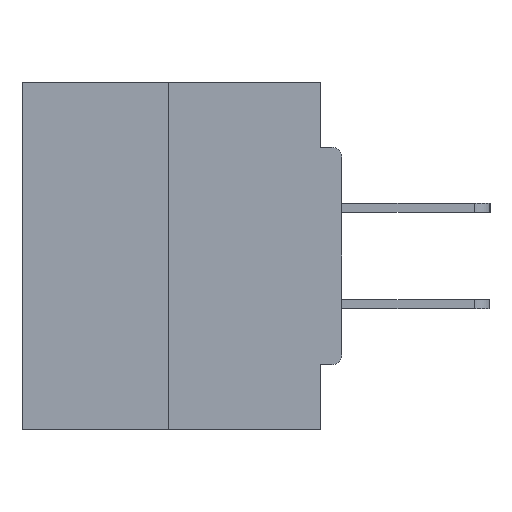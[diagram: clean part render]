
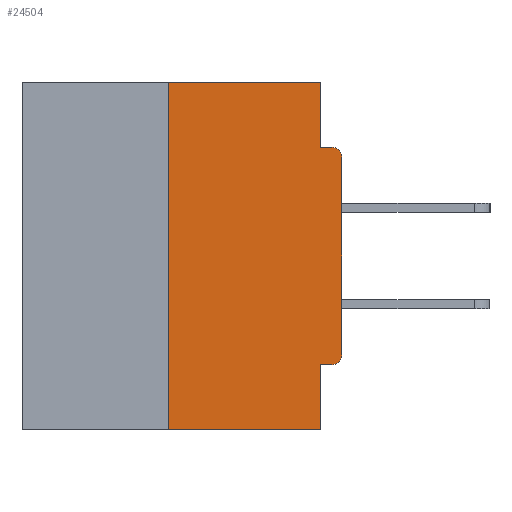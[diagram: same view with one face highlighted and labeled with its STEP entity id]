
A CAD part, left-side view. The second image highlights one B-rep face of the part: STEP entity #24504.
In plain terms, the highlighted planar face has unit normal (-1, 0, 0).
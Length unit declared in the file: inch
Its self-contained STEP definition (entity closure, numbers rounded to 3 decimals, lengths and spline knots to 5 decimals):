
#153 = LINE ( 'NONE', #21160, #10408 ) ;
#1027 = PLANE ( 'NONE',  #7817 ) ;
#1333 = CARTESIAN_POINT ( 'NONE',  ( 0., 0.031, -0.5 ) ) ;
#1667 = CIRCLE ( 'NONE', #7021, 0.015 ) ;
#2076 = CARTESIAN_POINT ( 'NONE',  ( 0., 0.25, -0.5 ) ) ;
#3086 = CARTESIAN_POINT ( 'NONE',  ( 0., 0., -0.3915 ) ) ;
#3103 = LINE ( 'NONE', #10801, #29433 ) ;
#3773 = ORIENTED_EDGE ( 'NONE', *, *, #5209, .T. ) ;
#3821 = CARTESIAN_POINT ( 'NONE',  ( 0., 0.46, 0. ) ) ;
#3864 = VECTOR ( 'NONE', #13528, 39.37008 ) ;
#5209 = EDGE_CURVE ( 'NONE', #28884, #12042, #21963, .T. ) ;
#6161 = LINE ( 'NONE', #11346, #18301 ) ;
#6567 = DIRECTION ( 'NONE',  ( 1., 0., 0. ) ) ;
#6850 = DIRECTION ( 'NONE',  ( 0., 0., -1. ) ) ;
#7021 = AXIS2_PLACEMENT_3D ( 'NONE', #30451, #27894, #24156 ) ;
#7236 = EDGE_LOOP ( 'NONE', ( #30805, #23453, #16780, #24602, #28934, #11545, #13261, #3773, #13718, #27101 ) ) ;
#7817 = AXIS2_PLACEMENT_3D ( 'NONE', #26764, #6567, #11266 ) ;
#7933 = VERTEX_POINT ( 'NONE', #22407 ) ;
#7979 = VERTEX_POINT ( 'NONE', #12443 ) ;
#8024 = CARTESIAN_POINT ( 'NONE',  ( 0., 0., -0.4065 ) ) ;
#8767 = DIRECTION ( 'NONE',  ( 0., -1., 0. ) ) ;
#9161 = EDGE_CURVE ( 'NONE', #17962, #7979, #15578, .T. ) ;
#9647 = CARTESIAN_POINT ( 'NONE',  ( 0., 0.015, -0.0935 ) ) ;
#10387 = VERTEX_POINT ( 'NONE', #16504 ) ;
#10408 = VECTOR ( 'NONE', #16284, 39.37008 ) ;
#10801 = CARTESIAN_POINT ( 'NONE',  ( 0., 0., 0. ) ) ;
#10902 = VECTOR ( 'NONE', #25854, 39.37008 ) ;
#11266 = DIRECTION ( 'NONE',  ( 0., 0., -1. ) ) ;
#11346 = CARTESIAN_POINT ( 'NONE',  ( 0., 0.031, -0.5 ) ) ;
#11534 = LINE ( 'NONE', #32125, #31478 ) ;
#11545 = ORIENTED_EDGE ( 'NONE', *, *, #21106, .T. ) ;
#11548 = EDGE_CURVE ( 'NONE', #10387, #7933, #11534, .T. ) ;
#12042 = VERTEX_POINT ( 'NONE', #9647 ) ;
#12443 = CARTESIAN_POINT ( 'NONE',  ( 0., 0.031, -0.4065 ) ) ;
#12738 = CARTESIAN_POINT ( 'NONE',  ( 0., 0.015, -0.4065 ) ) ;
#13010 = EDGE_CURVE ( 'NONE', #28650, #28884, #3103, .T. ) ;
#13261 = ORIENTED_EDGE ( 'NONE', *, *, #13010, .T. ) ;
#13321 = VERTEX_POINT ( 'NONE', #2076 ) ;
#13507 = CARTESIAN_POINT ( 'NONE',  ( 0., 0.25, 0. ) ) ;
#13528 = DIRECTION ( 'NONE',  ( 0., -1., 0. ) ) ;
#13718 = ORIENTED_EDGE ( 'NONE', *, *, #33293, .F. ) ;
#14375 = CARTESIAN_POINT ( 'NONE',  ( 0., 0.25, 0. ) ) ;
#15298 = CARTESIAN_POINT ( 'NONE',  ( 0., 0., -0.1085 ) ) ;
#15515 = AXIS2_PLACEMENT_3D ( 'NONE', #21858, #30284, #27744 ) ;
#15578 = LINE ( 'NONE', #8024, #10902 ) ;
#15834 = EDGE_CURVE ( 'NONE', #22573, #10387, #23640, .T. ) ;
#16058 = LINE ( 'NONE', #13507, #25382 ) ;
#16284 = DIRECTION ( 'NONE',  ( 0., -1., 0. ) ) ;
#16504 = CARTESIAN_POINT ( 'NONE',  ( 0., 0.031, 0. ) ) ;
#16667 = LINE ( 'NONE', #26276, #20945 ) ;
#16780 = ORIENTED_EDGE ( 'NONE', *, *, #27586, .T. ) ;
#17962 = VERTEX_POINT ( 'NONE', #12738 ) ;
#18301 = VECTOR ( 'NONE', #18614, 39.37008 ) ;
#18614 = DIRECTION ( 'NONE',  ( 0., 0., -1. ) ) ;
#20945 = VECTOR ( 'NONE', #8767, 39.37008 ) ;
#21073 = DIRECTION ( 'NONE',  ( 0., 0., 1. ) ) ;
#21106 = EDGE_CURVE ( 'NONE', #17962, #28650, #1667, .T. ) ;
#21150 = EDGE_CURVE ( 'NONE', #7979, #28185, #6161, .T. ) ;
#21160 = CARTESIAN_POINT ( 'NONE',  ( 0., 0., -0.0935 ) ) ;
#21858 = CARTESIAN_POINT ( 'NONE',  ( 0., 0.015, -0.1085 ) ) ;
#21963 = CIRCLE ( 'NONE', #15515, 0.015 ) ;
#22407 = CARTESIAN_POINT ( 'NONE',  ( 0., 0.031, -0.0935 ) ) ;
#22573 = VERTEX_POINT ( 'NONE', #14375 ) ;
#23453 = ORIENTED_EDGE ( 'NONE', *, *, #29966, .F. ) ;
#23640 = LINE ( 'NONE', #3821, #3864 ) ;
#24156 = DIRECTION ( 'NONE',  ( 0., 0., -1. ) ) ;
#24504 = ADVANCED_FACE ( 'NONE', ( #29651 ), #1027, .F. ) ;
#24602 = ORIENTED_EDGE ( 'NONE', *, *, #21150, .F. ) ;
#25382 = VECTOR ( 'NONE', #28873, 39.37008 ) ;
#25854 = DIRECTION ( 'NONE',  ( 0., 1., 0. ) ) ;
#26276 = CARTESIAN_POINT ( 'NONE',  ( 0., 0.46, -0.5 ) ) ;
#26764 = CARTESIAN_POINT ( 'NONE',  ( 0., 0.46, 0. ) ) ;
#27101 = ORIENTED_EDGE ( 'NONE', *, *, #11548, .F. ) ;
#27586 = EDGE_CURVE ( 'NONE', #13321, #28185, #16667, .T. ) ;
#27744 = DIRECTION ( 'NONE',  ( 0., 0., -1. ) ) ;
#27894 = DIRECTION ( 'NONE',  ( -1., 0., 0. ) ) ;
#28185 = VERTEX_POINT ( 'NONE', #1333 ) ;
#28650 = VERTEX_POINT ( 'NONE', #3086 ) ;
#28873 = DIRECTION ( 'NONE',  ( 0., 0., 1. ) ) ;
#28884 = VERTEX_POINT ( 'NONE', #15298 ) ;
#28934 = ORIENTED_EDGE ( 'NONE', *, *, #9161, .F. ) ;
#29433 = VECTOR ( 'NONE', #21073, 39.37008 ) ;
#29651 = FACE_OUTER_BOUND ( 'NONE', #7236, .T. ) ;
#29966 = EDGE_CURVE ( 'NONE', #13321, #22573, #16058, .T. ) ;
#30284 = DIRECTION ( 'NONE',  ( -1., 0., 0. ) ) ;
#30451 = CARTESIAN_POINT ( 'NONE',  ( 0., 0.015, -0.3915 ) ) ;
#30805 = ORIENTED_EDGE ( 'NONE', *, *, #15834, .F. ) ;
#31478 = VECTOR ( 'NONE', #6850, 39.37008 ) ;
#32125 = CARTESIAN_POINT ( 'NONE',  ( 0., 0.031, 0. ) ) ;
#33293 = EDGE_CURVE ( 'NONE', #7933, #12042, #153, .T. ) ;
